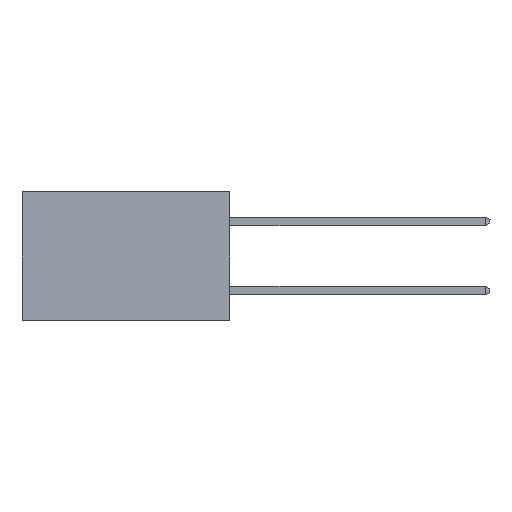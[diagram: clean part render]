
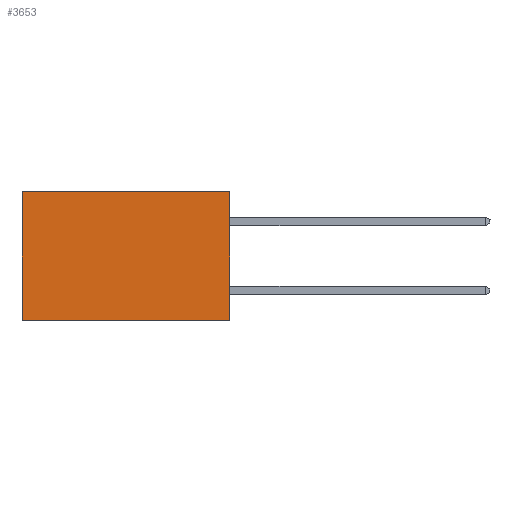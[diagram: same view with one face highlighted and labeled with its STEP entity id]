
A CAD part, left-side view. The second image highlights one B-rep face of the part: STEP entity #3653.
In plain terms, the highlighted planar face has unit normal (-1, 0, 0).
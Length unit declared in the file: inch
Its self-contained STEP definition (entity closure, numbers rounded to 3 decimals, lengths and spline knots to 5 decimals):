
#747 = ORIENTED_EDGE ( 'NONE', *, *, #4385, .T. ) ;
#935 = VECTOR ( 'NONE', #10726, 39.37008 ) ;
#1111 = FACE_OUTER_BOUND ( 'NONE', #15597, .T. ) ;
#1332 = CARTESIAN_POINT ( 'NONE',  ( 0.2615, 0., -0.37 ) ) ;
#3653 = ADVANCED_FACE ( 'NONE', ( #1111 ), #9245, .F. ) ;
#4031 = EDGE_CURVE ( 'NONE', #17876, #6609, #20967, .T. ) ;
#4385 = EDGE_CURVE ( 'NONE', #9437, #9172, #15912, .T. ) ;
#5140 = VECTOR ( 'NONE', #7100, 39.37008 ) ;
#5496 = CARTESIAN_POINT ( 'NONE',  ( 0.2615, 0.6, -0.37 ) ) ;
#5772 = CARTESIAN_POINT ( 'NONE',  ( 0.2615, 0., -0.37 ) ) ;
#5885 = VECTOR ( 'NONE', #14164, 39.37008 ) ;
#6609 = VERTEX_POINT ( 'NONE', #1332 ) ;
#7100 = DIRECTION ( 'NONE',  ( 0., 1., 0. ) ) ;
#8726 = LINE ( 'NONE', #11976, #5140 ) ;
#9172 = VERTEX_POINT ( 'NONE', #5496 ) ;
#9245 = PLANE ( 'NONE',  #13169 ) ;
#9437 = VERTEX_POINT ( 'NONE', #11243 ) ;
#9508 = CARTESIAN_POINT ( 'NONE',  ( 0.2615, 0.6, -0.37 ) ) ;
#9569 = VECTOR ( 'NONE', #10156, 39.37008 ) ;
#10156 = DIRECTION ( 'NONE',  ( 0., 1., 0. ) ) ;
#10726 = DIRECTION ( 'NONE',  ( 0., 0., -1. ) ) ;
#11191 = DIRECTION ( 'NONE',  ( 1., 0., 0. ) ) ;
#11243 = CARTESIAN_POINT ( 'NONE',  ( 0.2615, 0.6, 0. ) ) ;
#11647 = ORIENTED_EDGE ( 'NONE', *, *, #11939, .F. ) ;
#11939 = EDGE_CURVE ( 'NONE', #6609, #9172, #8726, .T. ) ;
#11976 = CARTESIAN_POINT ( 'NONE',  ( 0.2615, 0., -0.37 ) ) ;
#12927 = ORIENTED_EDGE ( 'NONE', *, *, #20164, .T. ) ;
#13169 = AXIS2_PLACEMENT_3D ( 'NONE', #5772, #11191, #20766 ) ;
#13991 = CARTESIAN_POINT ( 'NONE',  ( 0.2615, 0., -0.37 ) ) ;
#14164 = DIRECTION ( 'NONE',  ( 0., 0., -1. ) ) ;
#15597 = EDGE_LOOP ( 'NONE', ( #747, #11647, #19577, #12927 ) ) ;
#15912 = LINE ( 'NONE', #9508, #5885 ) ;
#16239 = CARTESIAN_POINT ( 'NONE',  ( 0.2615, 0., 0. ) ) ;
#17876 = VERTEX_POINT ( 'NONE', #19492 ) ;
#17884 = LINE ( 'NONE', #16239, #9569 ) ;
#19492 = CARTESIAN_POINT ( 'NONE',  ( 0.2615, 0., 0. ) ) ;
#19577 = ORIENTED_EDGE ( 'NONE', *, *, #4031, .F. ) ;
#20164 = EDGE_CURVE ( 'NONE', #17876, #9437, #17884, .T. ) ;
#20766 = DIRECTION ( 'NONE',  ( 0., 0., -1. ) ) ;
#20967 = LINE ( 'NONE', #13991, #935 ) ;
